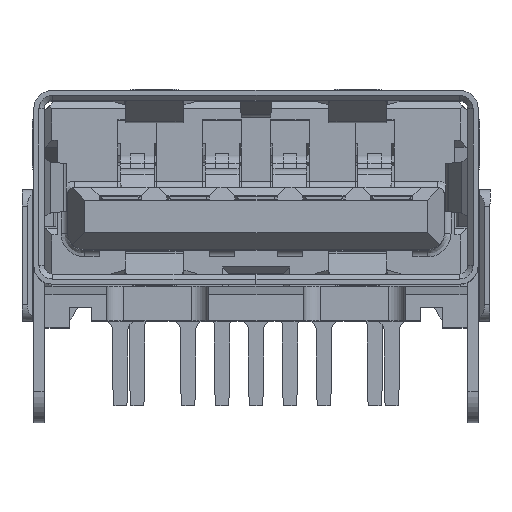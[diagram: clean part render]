
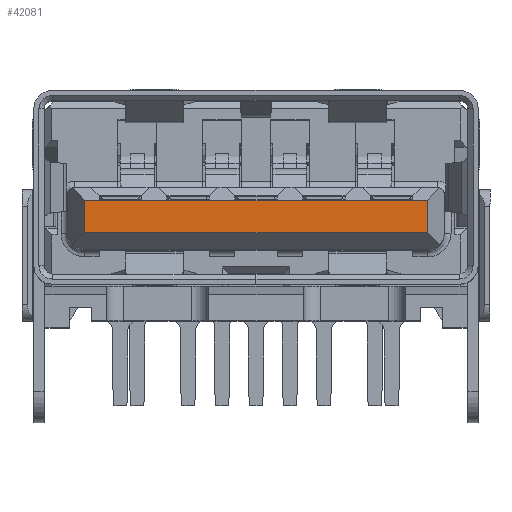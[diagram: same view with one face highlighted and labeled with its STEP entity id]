
A CAD part, top view. The second image highlights one B-rep face of the part: STEP entity #42081.
In plain terms, the highlighted face is planar.
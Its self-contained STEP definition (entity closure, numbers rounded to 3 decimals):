
#1900 = FACE_OUTER_BOUND ( 'NONE', #15910, .T. ) ;
#3933 = VERTEX_POINT ( 'NONE', #20091 ) ;
#5655 = VECTOR ( 'NONE', #28727, 1000. ) ;
#5725 = CARTESIAN_POINT ( 'NONE',  ( -30., -10.25, 0.38 ) ) ;
#6863 = DIRECTION ( 'NONE',  ( -1., 0., 0. ) ) ;
#8943 = LINE ( 'NONE', #9867, #5655 ) ;
#9867 = CARTESIAN_POINT ( 'NONE',  ( -24.95, -10.25, 0.86 ) ) ;
#15910 = EDGE_LOOP ( 'NONE', ( #28073, #48115, #25912, #26380 ) ) ;
#16774 = CARTESIAN_POINT ( 'NONE',  ( -24.748, -10.25, 1.365 ) ) ;
#17309 = LINE ( 'NONE', #41763, #53113 ) ;
#20091 = CARTESIAN_POINT ( 'NONE',  ( -24.95, -10.25, 1.34 ) ) ;
#20797 = PLANE ( 'NONE',  #25303 ) ;
#21446 = CARTESIAN_POINT ( 'NONE',  ( -35.05, -10.25, 0.38 ) ) ;
#22032 = EDGE_CURVE ( 'NONE', #37301, #57209, #44723, .T. ) ;
#22979 = EDGE_CURVE ( 'NONE', #3933, #31193, #59654, .T. ) ;
#23098 = CARTESIAN_POINT ( 'NONE',  ( -35.05, -10.25, 1.34 ) ) ;
#24619 = DIRECTION ( 'NONE',  ( 1., 0., 0. ) ) ;
#25303 = AXIS2_PLACEMENT_3D ( 'NONE', #16774, #58282, #6863 ) ;
#25912 = ORIENTED_EDGE ( 'NONE', *, *, #51664, .T. ) ;
#26380 = ORIENTED_EDGE ( 'NONE', *, *, #22979, .T. ) ;
#28073 = ORIENTED_EDGE ( 'NONE', *, *, #29191, .T. ) ;
#28727 = DIRECTION ( 'NONE',  ( 0., 0., 1. ) ) ;
#29191 = EDGE_CURVE ( 'NONE', #31193, #37301, #17309, .T. ) ;
#29414 = VECTOR ( 'NONE', #24619, 1000. ) ;
#31193 = VERTEX_POINT ( 'NONE', #23098 ) ;
#32046 = CARTESIAN_POINT ( 'NONE',  ( -30., -10.25, 1.34 ) ) ;
#37301 = VERTEX_POINT ( 'NONE', #21446 ) ;
#41763 = CARTESIAN_POINT ( 'NONE',  ( -35.05, -10.25, 0.86 ) ) ;
#42081 = ADVANCED_FACE ( 'NONE', ( #1900 ), #20797, .T. ) ;
#44723 = LINE ( 'NONE', #5725, #29414 ) ;
#46108 = DIRECTION ( 'NONE',  ( 0., 0., -1. ) ) ;
#48115 = ORIENTED_EDGE ( 'NONE', *, *, #22032, .T. ) ;
#50969 = DIRECTION ( 'NONE',  ( -1., 0., 0. ) ) ;
#51664 = EDGE_CURVE ( 'NONE', #57209, #3933, #8943, .T. ) ;
#53113 = VECTOR ( 'NONE', #46108, 1000. ) ;
#55804 = CARTESIAN_POINT ( 'NONE',  ( -24.95, -10.25, 0.38 ) ) ;
#57209 = VERTEX_POINT ( 'NONE', #55804 ) ;
#57224 = VECTOR ( 'NONE', #50969, 1000. ) ;
#58282 = DIRECTION ( 'NONE',  ( 0., -1., 0. ) ) ;
#59654 = LINE ( 'NONE', #32046, #57224 ) ;
